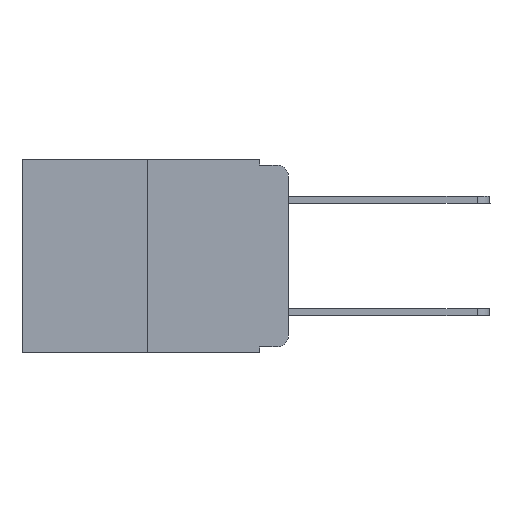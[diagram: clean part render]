
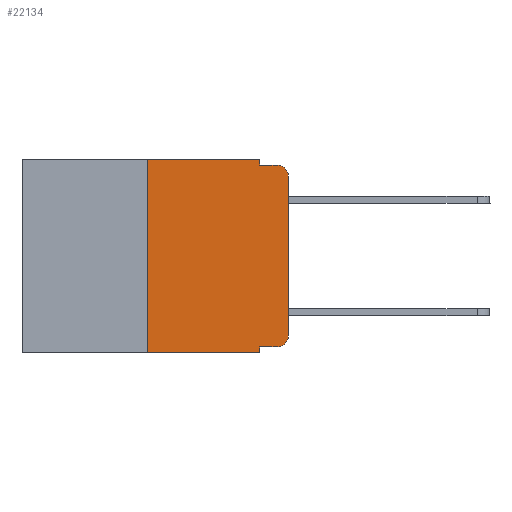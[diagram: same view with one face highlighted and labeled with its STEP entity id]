
A CAD part, left-side view. The second image highlights one B-rep face of the part: STEP entity #22134.
In plain terms, the highlighted planar face has unit normal (-1, 0, 0).
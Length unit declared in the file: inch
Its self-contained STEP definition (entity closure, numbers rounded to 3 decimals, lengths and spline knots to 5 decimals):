
#5 = PLANE ( 'NONE',  #8241 ) ;
#637 = CARTESIAN_POINT ( 'NONE',  ( 0., 0.25, -0.343 ) ) ;
#784 = VERTEX_POINT ( 'NONE', #13927 ) ;
#802 = LINE ( 'NONE', #18286, #18750 ) ;
#1477 = CARTESIAN_POINT ( 'NONE',  ( 0., 0.02, -0.01 ) ) ;
#1730 = CARTESIAN_POINT ( 'NONE',  ( 0., 0.051, -0.01 ) ) ;
#1970 = FACE_OUTER_BOUND ( 'NONE', #4556, .T. ) ;
#2244 = DIRECTION ( 'NONE',  ( 0., 0., -1. ) ) ;
#3751 = ORIENTED_EDGE ( 'NONE', *, *, #13769, .T. ) ;
#3849 = VERTEX_POINT ( 'NONE', #14421 ) ;
#4362 = CARTESIAN_POINT ( 'NONE',  ( 0., 0.051, -0.333 ) ) ;
#4556 = EDGE_LOOP ( 'NONE', ( #19942, #18414, #13047, #12957, #14271, #7947, #3751, #19708, #10941, #21523 ) ) ;
#4587 = VERTEX_POINT ( 'NONE', #14094 ) ;
#4972 = EDGE_CURVE ( 'NONE', #7877, #3849, #10007, .T. ) ;
#5010 = VERTEX_POINT ( 'NONE', #637 ) ;
#5485 = LINE ( 'NONE', #1730, #14992 ) ;
#6085 = EDGE_CURVE ( 'NONE', #784, #25320, #802, .T. ) ;
#6585 = EDGE_CURVE ( 'NONE', #12291, #784, #12533, .T. ) ;
#7068 = VECTOR ( 'NONE', #2244, 39.37008 ) ;
#7689 = DIRECTION ( 'NONE',  ( 0., 0., -1. ) ) ;
#7877 = VERTEX_POINT ( 'NONE', #11676 ) ;
#7947 = ORIENTED_EDGE ( 'NONE', *, *, #10673, .F. ) ;
#8133 = CARTESIAN_POINT ( 'NONE',  ( 0., 0.02, -0.313 ) ) ;
#8241 = AXIS2_PLACEMENT_3D ( 'NONE', #10503, #15178, #10778 ) ;
#8865 = DIRECTION ( 'NONE',  ( 0., -1., 0. ) ) ;
#9160 = VERTEX_POINT ( 'NONE', #1477 ) ;
#10007 = LINE ( 'NONE', #21084, #16882 ) ;
#10148 = DIRECTION ( 'NONE',  ( 0., 0., 1. ) ) ;
#10298 = DIRECTION ( 'NONE',  ( 0., -1., 0. ) ) ;
#10373 = EDGE_CURVE ( 'NONE', #21833, #9160, #5485, .T. ) ;
#10385 = DIRECTION ( 'NONE',  ( 0., 0., -1. ) ) ;
#10503 = CARTESIAN_POINT ( 'NONE',  ( 0., 0.473, 0. ) ) ;
#10673 = EDGE_CURVE ( 'NONE', #5010, #7877, #22996, .T. ) ;
#10778 = DIRECTION ( 'NONE',  ( 0., 0., -1. ) ) ;
#10805 = CARTESIAN_POINT ( 'NONE',  ( 0., 0.02, -0.333 ) ) ;
#10911 = CARTESIAN_POINT ( 'NONE',  ( 0., 0.051, 0. ) ) ;
#10941 = ORIENTED_EDGE ( 'NONE', *, *, #16623, .T. ) ;
#11630 = LINE ( 'NONE', #4362, #15861 ) ;
#11676 = CARTESIAN_POINT ( 'NONE',  ( 0., 0.25, 0. ) ) ;
#11865 = CARTESIAN_POINT ( 'NONE',  ( 0., 0.051, 0. ) ) ;
#12175 = CARTESIAN_POINT ( 'NONE',  ( 0., 0.25, 0. ) ) ;
#12291 = VERTEX_POINT ( 'NONE', #10805 ) ;
#12409 = CARTESIAN_POINT ( 'NONE',  ( 0., 0.02, -0.03 ) ) ;
#12533 = CIRCLE ( 'NONE', #22991, 0.02 ) ;
#12957 = ORIENTED_EDGE ( 'NONE', *, *, #26535, .F. ) ;
#13047 = ORIENTED_EDGE ( 'NONE', *, *, #10373, .F. ) ;
#13769 = EDGE_CURVE ( 'NONE', #5010, #18189, #14074, .T. ) ;
#13927 = CARTESIAN_POINT ( 'NONE',  ( 0., 0., -0.313 ) ) ;
#14074 = LINE ( 'NONE', #15287, #26741 ) ;
#14094 = CARTESIAN_POINT ( 'NONE',  ( 0., 0.051, -0.333 ) ) ;
#14220 = DIRECTION ( 'NONE',  ( 0., 0., 1. ) ) ;
#14271 = ORIENTED_EDGE ( 'NONE', *, *, #4972, .F. ) ;
#14421 = CARTESIAN_POINT ( 'NONE',  ( 0., 0.051, 0. ) ) ;
#14992 = VECTOR ( 'NONE', #8865, 39.37008 ) ;
#15178 = DIRECTION ( 'NONE',  ( 1., 0., 0. ) ) ;
#15287 = CARTESIAN_POINT ( 'NONE',  ( 0., 0.473, -0.343 ) ) ;
#15861 = VECTOR ( 'NONE', #10298, 39.37008 ) ;
#16198 = CIRCLE ( 'NONE', #21432, 0.02 ) ;
#16623 = EDGE_CURVE ( 'NONE', #4587, #12291, #11630, .T. ) ;
#16882 = VECTOR ( 'NONE', #17169, 39.37008 ) ;
#17169 = DIRECTION ( 'NONE',  ( 0., -1., 0. ) ) ;
#18096 = CARTESIAN_POINT ( 'NONE',  ( 0., 0.051, -0.343 ) ) ;
#18189 = VERTEX_POINT ( 'NONE', #18096 ) ;
#18286 = CARTESIAN_POINT ( 'NONE',  ( 0., 0., 0. ) ) ;
#18414 = ORIENTED_EDGE ( 'NONE', *, *, #23395, .T. ) ;
#18420 = DIRECTION ( 'NONE',  ( -1., 0., 0. ) ) ;
#18750 = VECTOR ( 'NONE', #14220, 39.37008 ) ;
#19708 = ORIENTED_EDGE ( 'NONE', *, *, #20269, .F. ) ;
#19942 = ORIENTED_EDGE ( 'NONE', *, *, #6085, .T. ) ;
#20269 = EDGE_CURVE ( 'NONE', #4587, #18189, #25617, .T. ) ;
#20296 = VECTOR ( 'NONE', #10148, 39.37008 ) ;
#21084 = CARTESIAN_POINT ( 'NONE',  ( 0., 0.473, 0. ) ) ;
#21432 = AXIS2_PLACEMENT_3D ( 'NONE', #12409, #18420, #10385 ) ;
#21523 = ORIENTED_EDGE ( 'NONE', *, *, #6585, .T. ) ;
#21662 = DIRECTION ( 'NONE',  ( 0., -1., 0. ) ) ;
#21751 = LINE ( 'NONE', #10911, #7068 ) ;
#21833 = VERTEX_POINT ( 'NONE', #25774 ) ;
#22134 = ADVANCED_FACE ( 'NONE', ( #1970 ), #5, .F. ) ;
#22836 = CARTESIAN_POINT ( 'NONE',  ( 0., 0., -0.03 ) ) ;
#22991 = AXIS2_PLACEMENT_3D ( 'NONE', #8133, #26469, #7689 ) ;
#22996 = LINE ( 'NONE', #12175, #20296 ) ;
#23395 = EDGE_CURVE ( 'NONE', #25320, #9160, #16198, .T. ) ;
#25320 = VERTEX_POINT ( 'NONE', #22836 ) ;
#25617 = LINE ( 'NONE', #11865, #25949 ) ;
#25774 = CARTESIAN_POINT ( 'NONE',  ( 0., 0.051, -0.01 ) ) ;
#25949 = VECTOR ( 'NONE', #26541, 39.37008 ) ;
#26469 = DIRECTION ( 'NONE',  ( -1., 0., 0. ) ) ;
#26535 = EDGE_CURVE ( 'NONE', #3849, #21833, #21751, .T. ) ;
#26541 = DIRECTION ( 'NONE',  ( 0., 0., -1. ) ) ;
#26741 = VECTOR ( 'NONE', #21662, 39.37008 ) ;
